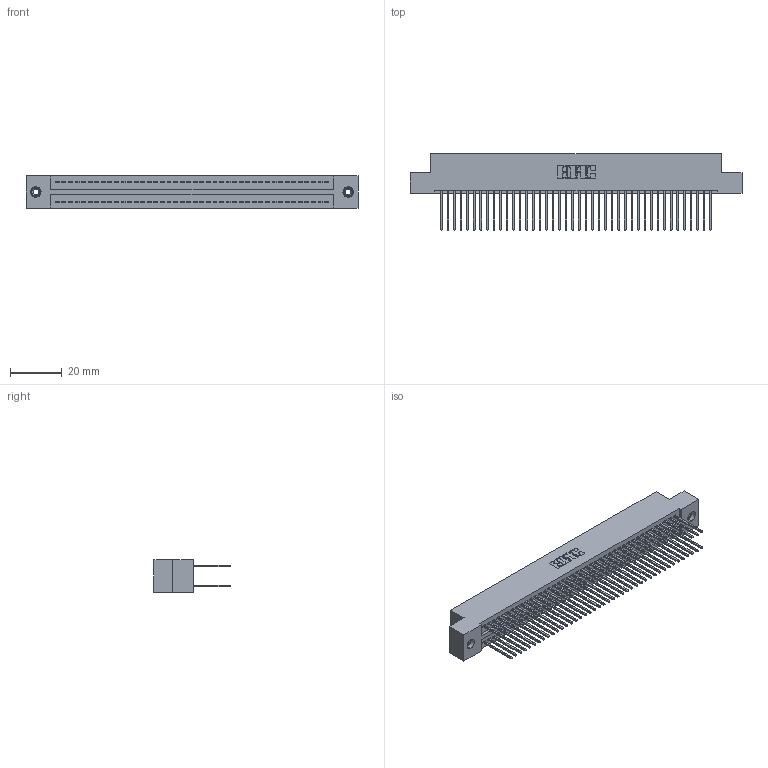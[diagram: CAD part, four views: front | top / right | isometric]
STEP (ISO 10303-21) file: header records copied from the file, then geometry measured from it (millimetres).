
FILE_DESCRIPTION (( 'STEP AP203' ), '1' );
FILE_NAME ('325-084-540-208.STEP', '2020-02-25T05:07:06', ( '' ), ( '' ), 'SwSTEP 2.0', 'SolidWorks 2016', '' );
FILE_SCHEMA (( 'CONFIG_CONTROL_DESIGN' ));
Length unit declared in the file: inch
Products named in the file (4): 325-292-001_325-293-140; 325-084-540-208; 345-250-001_345-250-003-102; 325 Part_TI
Assembly tree (87 placements, depth 2):
  325-084-540-208
    325 Part_TI
    325-292-001_325-293-140  x84
    345-250-001_345-250-003-102  x2
Bounding box: 128.4 x 29.46 x 12.45 mm (x, y, z)
Volume: 16887.6 mm3; surface area: 21969.7 mm2
Topology: 87 solids, 87 shells, 4542 faces, 13467 edges, 8858 vertices
Faces by surface type: plane 3126, cylinder 1400, cone 12, torus 4
Entity records: 28224 total; most frequent: CARTESIAN_POINT 4661, ORIENTED_EDGE 4590, DIRECTION 4013, EDGE_CURVE 2295, VECTOR 2147, LINE 2147, VERTEX_POINT 1524, AXIS2_PLACEMENT_3D 933
